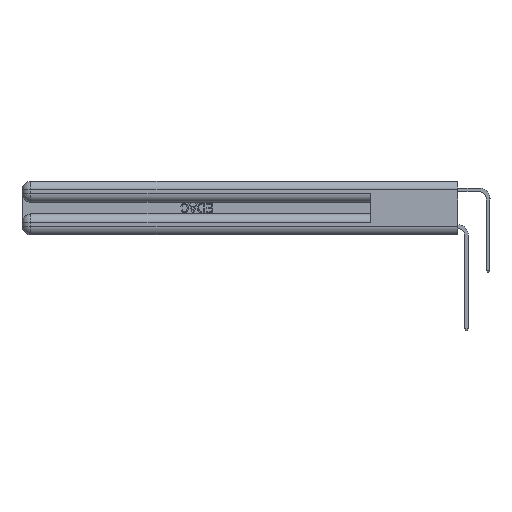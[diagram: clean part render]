
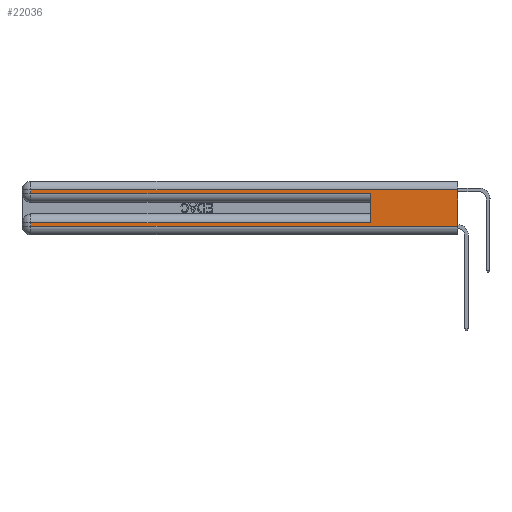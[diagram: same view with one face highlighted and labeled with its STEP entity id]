
A CAD part, left-side view. The second image highlights one B-rep face of the part: STEP entity #22036.
In plain terms, the highlighted planar face has unit normal (-1, 0, 0).
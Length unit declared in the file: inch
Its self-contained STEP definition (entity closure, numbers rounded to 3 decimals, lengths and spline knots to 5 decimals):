
#1302 = LINE ( 'NONE', #21607, #25326 ) ;
#1911 = LINE ( 'NONE', #10022, #18175 ) ;
#1913 = EDGE_CURVE ( 'NONE', #16433, #23772, #1911, .T. ) ;
#2030 = ORIENTED_EDGE ( 'NONE', *, *, #22660, .F. ) ;
#2576 = LINE ( 'NONE', #28006, #25865 ) ;
#3075 = EDGE_CURVE ( 'NONE', #16461, #11308, #2576, .T. ) ;
#3307 = LINE ( 'NONE', #8576, #20643 ) ;
#4268 = CARTESIAN_POINT ( 'NONE',  ( 0., 2.94, 0.285 ) ) ;
#4588 = CARTESIAN_POINT ( 'NONE',  ( 0., 0., 0.37 ) ) ;
#5781 = ORIENTED_EDGE ( 'NONE', *, *, #27962, .T. ) ;
#5856 = CARTESIAN_POINT ( 'NONE',  ( 0., 2.94, 0.085 ) ) ;
#6136 = LINE ( 'NONE', #17620, #20633 ) ;
#6181 = DIRECTION ( 'NONE',  ( 0., 0., -1. ) ) ;
#6765 = EDGE_CURVE ( 'NONE', #11308, #22742, #20482, .T. ) ;
#7267 = VECTOR ( 'NONE', #9668, 39.37008 ) ;
#8329 = DIRECTION ( 'NONE',  ( 0., 1., 0. ) ) ;
#8576 = CARTESIAN_POINT ( 'NONE',  ( 0., 0.6, 0.145 ) ) ;
#8808 = PLANE ( 'NONE',  #14887 ) ;
#9241 = CARTESIAN_POINT ( 'NONE',  ( 0., 0.6, 0.285 ) ) ;
#9382 = VERTEX_POINT ( 'NONE', #5856 ) ;
#9622 = EDGE_CURVE ( 'NONE', #9382, #16433, #6136, .T. ) ;
#9668 = DIRECTION ( 'NONE',  ( 0., 0., -1. ) ) ;
#10022 = CARTESIAN_POINT ( 'NONE',  ( 0., 0., 0.06 ) ) ;
#10135 = ORIENTED_EDGE ( 'NONE', *, *, #9622, .T. ) ;
#10583 = ORIENTED_EDGE ( 'NONE', *, *, #6765, .T. ) ;
#10955 = DIRECTION ( 'NONE',  ( 0., 0., 1. ) ) ;
#11308 = VERTEX_POINT ( 'NONE', #4268 ) ;
#11516 = CARTESIAN_POINT ( 'NONE',  ( 0., 0., 0.285 ) ) ;
#11558 = ORIENTED_EDGE ( 'NONE', *, *, #3075, .T. ) ;
#11562 = DIRECTION ( 'NONE',  ( 0., 1., 0. ) ) ;
#11615 = DIRECTION ( 'NONE',  ( 0., -1., 0. ) ) ;
#13338 = ORIENTED_EDGE ( 'NONE', *, *, #15869, .T. ) ;
#13769 = CARTESIAN_POINT ( 'NONE',  ( 0., 0.6, 0.085 ) ) ;
#14887 = AXIS2_PLACEMENT_3D ( 'NONE', #15547, #24622, #18195 ) ;
#15547 = CARTESIAN_POINT ( 'NONE',  ( 0., 0., 0.37 ) ) ;
#15869 = EDGE_CURVE ( 'NONE', #28083, #16461, #22501, .T. ) ;
#16433 = VERTEX_POINT ( 'NONE', #26619 ) ;
#16461 = VERTEX_POINT ( 'NONE', #18501 ) ;
#17510 = VECTOR ( 'NONE', #11562, 39.37008 ) ;
#17620 = CARTESIAN_POINT ( 'NONE',  ( 0., 2.94, 0.37 ) ) ;
#18175 = VECTOR ( 'NONE', #23699, 39.37008 ) ;
#18195 = DIRECTION ( 'NONE',  ( 0., 0., -1. ) ) ;
#18501 = CARTESIAN_POINT ( 'NONE',  ( 0., 2.94, 0.31 ) ) ;
#18759 = DIRECTION ( 'NONE',  ( 0., 0., -1. ) ) ;
#19980 = ORIENTED_EDGE ( 'NONE', *, *, #1913, .T. ) ;
#20432 = VERTEX_POINT ( 'NONE', #13769 ) ;
#20482 = LINE ( 'NONE', #11516, #27464 ) ;
#20633 = VECTOR ( 'NONE', #6181, 39.37008 ) ;
#20643 = VECTOR ( 'NONE', #10955, 39.37008 ) ;
#20833 = EDGE_CURVE ( 'NONE', #28083, #23772, #27038, .T. ) ;
#21607 = CARTESIAN_POINT ( 'NONE',  ( 0., 0., 0.085 ) ) ;
#22036 = ADVANCED_FACE ( 'NONE', ( #27318 ), #8808, .F. ) ;
#22501 = LINE ( 'NONE', #25090, #17510 ) ;
#22660 = EDGE_CURVE ( 'NONE', #20432, #22742, #3307, .T. ) ;
#22742 = VERTEX_POINT ( 'NONE', #9241 ) ;
#23699 = DIRECTION ( 'NONE',  ( 0., -1., 0. ) ) ;
#23772 = VERTEX_POINT ( 'NONE', #23858 ) ;
#23858 = CARTESIAN_POINT ( 'NONE',  ( 0., 0., 0.06 ) ) ;
#24243 = EDGE_LOOP ( 'NONE', ( #26024, #13338, #11558, #10583, #2030, #5781, #10135, #19980 ) ) ;
#24622 = DIRECTION ( 'NONE',  ( 1., 0., 0. ) ) ;
#25090 = CARTESIAN_POINT ( 'NONE',  ( 0., 0., 0.31 ) ) ;
#25326 = VECTOR ( 'NONE', #8329, 39.37008 ) ;
#25865 = VECTOR ( 'NONE', #18759, 39.37008 ) ;
#26024 = ORIENTED_EDGE ( 'NONE', *, *, #20833, .F. ) ;
#26619 = CARTESIAN_POINT ( 'NONE',  ( 0., 2.94, 0.06 ) ) ;
#27038 = LINE ( 'NONE', #4588, #7267 ) ;
#27318 = FACE_OUTER_BOUND ( 'NONE', #24243, .T. ) ;
#27464 = VECTOR ( 'NONE', #11615, 39.37008 ) ;
#27962 = EDGE_CURVE ( 'NONE', #20432, #9382, #1302, .T. ) ;
#28006 = CARTESIAN_POINT ( 'NONE',  ( 0., 2.94, 0.37 ) ) ;
#28083 = VERTEX_POINT ( 'NONE', #28366 ) ;
#28366 = CARTESIAN_POINT ( 'NONE',  ( 0., 0., 0.31 ) ) ;
